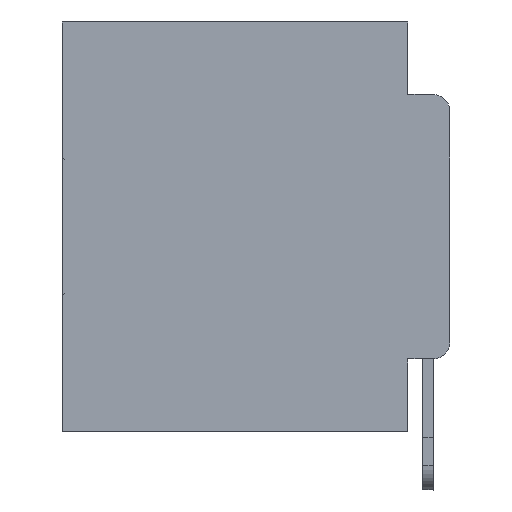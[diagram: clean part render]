
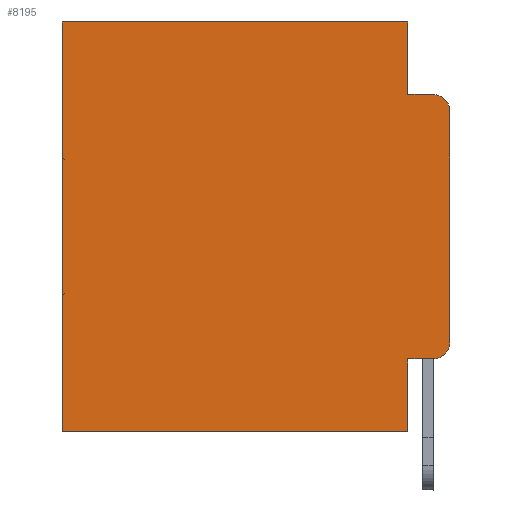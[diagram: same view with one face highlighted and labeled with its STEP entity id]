
A CAD part, left-side view. The second image highlights one B-rep face of the part: STEP entity #8195.
In plain terms, the highlighted planar face has unit normal (-1, 0, 0).
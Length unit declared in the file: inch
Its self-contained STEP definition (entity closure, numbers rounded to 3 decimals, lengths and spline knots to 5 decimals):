
#148 = LINE ( 'NONE', #25453, #24470 ) ;
#394 = CARTESIAN_POINT ( 'NONE',  ( 0.298, 0.051, 0. ) ) ;
#465 = CARTESIAN_POINT ( 'NONE',  ( 0.298, 0.473, 0. ) ) ;
#640 = VECTOR ( 'NONE', #9494, 39.37008 ) ;
#879 = CIRCLE ( 'NONE', #4394, 0.02 ) ;
#1862 = EDGE_CURVE ( 'NONE', #12607, #2630, #18550, .T. ) ;
#2159 = CARTESIAN_POINT ( 'NONE',  ( 0.298, 0., 0. ) ) ;
#2593 = DIRECTION ( 'NONE',  ( 0., 0., -1. ) ) ;
#2630 = VERTEX_POINT ( 'NONE', #22026 ) ;
#2666 = ORIENTED_EDGE ( 'NONE', *, *, #27778, .T. ) ;
#3321 = VECTOR ( 'NONE', #23026, 39.37008 ) ;
#3604 = VERTEX_POINT ( 'NONE', #13224 ) ;
#3743 = EDGE_CURVE ( 'NONE', #11717, #17161, #29582, .T. ) ;
#4394 = AXIS2_PLACEMENT_3D ( 'NONE', #29049, #14672, #2593 ) ;
#5456 = EDGE_CURVE ( 'NONE', #17895, #14277, #148, .T. ) ;
#5511 = CARTESIAN_POINT ( 'NONE',  ( 0.298, 0.473, 0. ) ) ;
#6338 = LINE ( 'NONE', #21919, #20300 ) ;
#6369 = LINE ( 'NONE', #10715, #3321 ) ;
#6454 = CARTESIAN_POINT ( 'NONE',  ( 0.298, 0., 0. ) ) ;
#6866 = ORIENTED_EDGE ( 'NONE', *, *, #14399, .F. ) ;
#7034 = ORIENTED_EDGE ( 'NONE', *, *, #19618, .F. ) ;
#8137 = ORIENTED_EDGE ( 'NONE', *, *, #14943, .T. ) ;
#8195 = ADVANCED_FACE ( 'NONE', ( #8343 ), #18293, .F. ) ;
#8343 = FACE_OUTER_BOUND ( 'NONE', #25342, .T. ) ;
#8896 = DIRECTION ( 'NONE',  ( 0., 1., 0. ) ) ;
#9204 = DIRECTION ( 'NONE',  ( 1., 0., 0. ) ) ;
#9465 = LINE ( 'NONE', #17405, #16644 ) ;
#9494 = DIRECTION ( 'NONE',  ( 0., 0., -1. ) ) ;
#10106 = CARTESIAN_POINT ( 'NONE',  ( 0.298, 0.051, -0.4115 ) ) ;
#10159 = DIRECTION ( 'NONE',  ( 0., 0., -1. ) ) ;
#10347 = CIRCLE ( 'NONE', #12264, 0.02 ) ;
#10715 = CARTESIAN_POINT ( 'NONE',  ( 0.298, 0.051, 0. ) ) ;
#11717 = VERTEX_POINT ( 'NONE', #394 ) ;
#12195 = DIRECTION ( 'NONE',  ( 0., 1., 0. ) ) ;
#12234 = ORIENTED_EDGE ( 'NONE', *, *, #1862, .F. ) ;
#12264 = AXIS2_PLACEMENT_3D ( 'NONE', #12874, #27766, #17749 ) ;
#12607 = VERTEX_POINT ( 'NONE', #25423 ) ;
#12874 = CARTESIAN_POINT ( 'NONE',  ( 0.298, 0.02, -0.3915 ) ) ;
#13224 = CARTESIAN_POINT ( 'NONE',  ( 0.298, 0.02, -0.4115 ) ) ;
#13252 = ORIENTED_EDGE ( 'NONE', *, *, #3743, .T. ) ;
#13331 = DIRECTION ( 'NONE',  ( 0., -1., 0. ) ) ;
#14277 = VERTEX_POINT ( 'NONE', #17703 ) ;
#14399 = EDGE_CURVE ( 'NONE', #11717, #17895, #6369, .T. ) ;
#14672 = DIRECTION ( 'NONE',  ( -1., 0., 0. ) ) ;
#14943 = EDGE_CURVE ( 'NONE', #17161, #2630, #19209, .T. ) ;
#15761 = ORIENTED_EDGE ( 'NONE', *, *, #21205, .F. ) ;
#16014 = CARTESIAN_POINT ( 'NONE',  ( 0.298, 0., -0.1085 ) ) ;
#16173 = LINE ( 'NONE', #2159, #640 ) ;
#16644 = VECTOR ( 'NONE', #27845, 39.37008 ) ;
#17161 = VERTEX_POINT ( 'NONE', #465 ) ;
#17405 = CARTESIAN_POINT ( 'NONE',  ( 0.298, 0.051, 0. ) ) ;
#17497 = EDGE_CURVE ( 'NONE', #23926, #14277, #879, .T. ) ;
#17703 = CARTESIAN_POINT ( 'NONE',  ( 0.298, 0.02, -0.0885 ) ) ;
#17749 = DIRECTION ( 'NONE',  ( 0., 0., -1. ) ) ;
#17895 = VERTEX_POINT ( 'NONE', #18748 ) ;
#18202 = ORIENTED_EDGE ( 'NONE', *, *, #30140, .T. ) ;
#18293 = PLANE ( 'NONE',  #18369 ) ;
#18369 = AXIS2_PLACEMENT_3D ( 'NONE', #25665, #9204, #23624 ) ;
#18550 = LINE ( 'NONE', #26778, #28482 ) ;
#18748 = CARTESIAN_POINT ( 'NONE',  ( 0.298, 0.051, -0.0885 ) ) ;
#19209 = LINE ( 'NONE', #5511, #31480 ) ;
#19618 = EDGE_CURVE ( 'NONE', #30658, #12607, #9465, .T. ) ;
#20300 = VECTOR ( 'NONE', #22350, 39.37008 ) ;
#21205 = EDGE_CURVE ( 'NONE', #23926, #27409, #16173, .T. ) ;
#21919 = CARTESIAN_POINT ( 'NONE',  ( 0.298, 0.051, -0.4115 ) ) ;
#22026 = CARTESIAN_POINT ( 'NONE',  ( 0.298, 0.473, -0.5 ) ) ;
#22309 = ORIENTED_EDGE ( 'NONE', *, *, #5456, .F. ) ;
#22350 = DIRECTION ( 'NONE',  ( 0., -1., 0. ) ) ;
#23026 = DIRECTION ( 'NONE',  ( 0., 0., -1. ) ) ;
#23624 = DIRECTION ( 'NONE',  ( 0., 0., -1. ) ) ;
#23844 = VECTOR ( 'NONE', #8896, 39.37008 ) ;
#23926 = VERTEX_POINT ( 'NONE', #16014 ) ;
#24458 = ORIENTED_EDGE ( 'NONE', *, *, #17497, .T. ) ;
#24470 = VECTOR ( 'NONE', #13331, 39.37008 ) ;
#25342 = EDGE_LOOP ( 'NONE', ( #15761, #24458, #22309, #6866, #13252, #8137, #12234, #7034, #2666, #18202 ) ) ;
#25423 = CARTESIAN_POINT ( 'NONE',  ( 0.298, 0.051, -0.5 ) ) ;
#25453 = CARTESIAN_POINT ( 'NONE',  ( 0.298, 0.051, -0.0885 ) ) ;
#25665 = CARTESIAN_POINT ( 'NONE',  ( 0.298, 0., 0. ) ) ;
#26778 = CARTESIAN_POINT ( 'NONE',  ( 0.298, 0., -0.5 ) ) ;
#27409 = VERTEX_POINT ( 'NONE', #27936 ) ;
#27766 = DIRECTION ( 'NONE',  ( -1., 0., 0. ) ) ;
#27778 = EDGE_CURVE ( 'NONE', #30658, #3604, #6338, .T. ) ;
#27845 = DIRECTION ( 'NONE',  ( 0., 0., -1. ) ) ;
#27936 = CARTESIAN_POINT ( 'NONE',  ( 0.298, 0., -0.3915 ) ) ;
#28482 = VECTOR ( 'NONE', #12195, 39.37008 ) ;
#29049 = CARTESIAN_POINT ( 'NONE',  ( 0.298, 0.02, -0.1085 ) ) ;
#29582 = LINE ( 'NONE', #6454, #23844 ) ;
#30140 = EDGE_CURVE ( 'NONE', #3604, #27409, #10347, .T. ) ;
#30658 = VERTEX_POINT ( 'NONE', #10106 ) ;
#31480 = VECTOR ( 'NONE', #10159, 39.37008 ) ;
